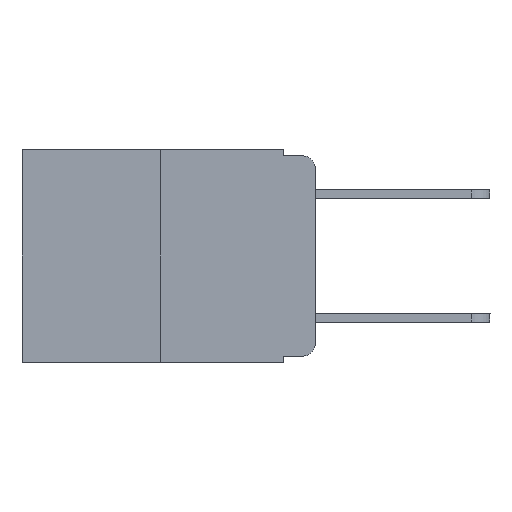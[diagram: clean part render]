
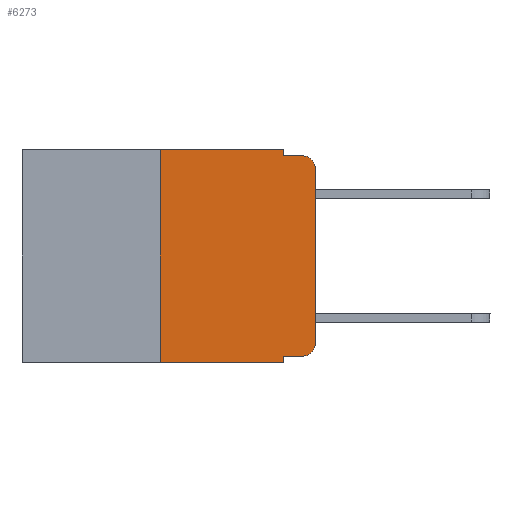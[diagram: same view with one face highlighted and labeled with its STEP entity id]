
A CAD part, left-side view. The second image highlights one B-rep face of the part: STEP entity #6273.
In plain terms, the highlighted planar face has unit normal (-1, 0, 0).
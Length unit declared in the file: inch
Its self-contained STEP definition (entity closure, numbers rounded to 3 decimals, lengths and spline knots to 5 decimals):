
#182 = CIRCLE ( 'NONE', #10225, 0.02 ) ;
#445 = CARTESIAN_POINT ( 'NONE',  ( 0., 0.051, -0.333 ) ) ;
#484 = VERTEX_POINT ( 'NONE', #7093 ) ;
#715 = CARTESIAN_POINT ( 'NONE',  ( 0., 0.051, 0. ) ) ;
#750 = ORIENTED_EDGE ( 'NONE', *, *, #6286, .T. ) ;
#757 = VERTEX_POINT ( 'NONE', #15017 ) ;
#823 = LINE ( 'NONE', #2420, #1748 ) ;
#1157 = DIRECTION ( 'NONE',  ( -1., 0., 0. ) ) ;
#1341 = ORIENTED_EDGE ( 'NONE', *, *, #10828, .T. ) ;
#1599 = ORIENTED_EDGE ( 'NONE', *, *, #10114, .F. ) ;
#1748 = VECTOR ( 'NONE', #13231, 39.37008 ) ;
#1976 = VECTOR ( 'NONE', #14798, 39.37008 ) ;
#2177 = CIRCLE ( 'NONE', #5035, 0.02 ) ;
#2183 = DIRECTION ( 'NONE',  ( 0., -1., 0. ) ) ;
#2420 = CARTESIAN_POINT ( 'NONE',  ( 0., 0.473, 0. ) ) ;
#2553 = LINE ( 'NONE', #9236, #14938 ) ;
#2560 = CARTESIAN_POINT ( 'NONE',  ( 0., 0., -0.03 ) ) ;
#2657 = VERTEX_POINT ( 'NONE', #14166 ) ;
#2874 = VERTEX_POINT ( 'NONE', #9908 ) ;
#3619 = ORIENTED_EDGE ( 'NONE', *, *, #7371, .F. ) ;
#3761 = CARTESIAN_POINT ( 'NONE',  ( 0., 0., 0. ) ) ;
#3786 = CARTESIAN_POINT ( 'NONE',  ( 0., 0.051, -0.01 ) ) ;
#4006 = CARTESIAN_POINT ( 'NONE',  ( 0., 0.051, -0.333 ) ) ;
#4274 = EDGE_LOOP ( 'NONE', ( #11995, #1341, #12284, #1599, #7026, #13450, #15163, #3619, #6871, #750 ) ) ;
#4278 = CARTESIAN_POINT ( 'NONE',  ( 0., 0.25, 0. ) ) ;
#4734 = PLANE ( 'NONE',  #6441 ) ;
#5035 = AXIS2_PLACEMENT_3D ( 'NONE', #5893, #5844, #8236 ) ;
#5484 = DIRECTION ( 'NONE',  ( 0., 0., 1. ) ) ;
#5844 = DIRECTION ( 'NONE',  ( -1., 0., 0. ) ) ;
#5893 = CARTESIAN_POINT ( 'NONE',  ( 0., 0.02, -0.313 ) ) ;
#5907 = LINE ( 'NONE', #445, #1976 ) ;
#6107 = VERTEX_POINT ( 'NONE', #4006 ) ;
#6273 = ADVANCED_FACE ( 'NONE', ( #10043 ), #4734, .F. ) ;
#6286 = EDGE_CURVE ( 'NONE', #10520, #2874, #2177, .T. ) ;
#6420 = LINE ( 'NONE', #3761, #13572 ) ;
#6441 = AXIS2_PLACEMENT_3D ( 'NONE', #13153, #12944, #12999 ) ;
#6871 = ORIENTED_EDGE ( 'NONE', *, *, #7789, .T. ) ;
#7026 = ORIENTED_EDGE ( 'NONE', *, *, #9501, .F. ) ;
#7093 = CARTESIAN_POINT ( 'NONE',  ( 0., 0.25, 0. ) ) ;
#7371 = EDGE_CURVE ( 'NONE', #6107, #757, #2553, .T. ) ;
#7789 = EDGE_CURVE ( 'NONE', #6107, #10520, #5907, .T. ) ;
#8124 = DIRECTION ( 'NONE',  ( 0., 0., -1. ) ) ;
#8236 = DIRECTION ( 'NONE',  ( 0., 0., -1. ) ) ;
#8783 = CARTESIAN_POINT ( 'NONE',  ( 0., 0.25, -0.343 ) ) ;
#9236 = CARTESIAN_POINT ( 'NONE',  ( 0., 0.051, 0. ) ) ;
#9501 = EDGE_CURVE ( 'NONE', #484, #14658, #823, .T. ) ;
#9786 = DIRECTION ( 'NONE',  ( 0., -1., 0. ) ) ;
#9908 = CARTESIAN_POINT ( 'NONE',  ( 0., 0., -0.313 ) ) ;
#9984 = EDGE_CURVE ( 'NONE', #15344, #484, #9996, .T. ) ;
#9996 = LINE ( 'NONE', #4278, #13950 ) ;
#10043 = FACE_OUTER_BOUND ( 'NONE', #4274, .T. ) ;
#10114 = EDGE_CURVE ( 'NONE', #14658, #11758, #15314, .T. ) ;
#10225 = AXIS2_PLACEMENT_3D ( 'NONE', #12977, #1157, #13076 ) ;
#10361 = EDGE_CURVE ( 'NONE', #15344, #757, #11421, .T. ) ;
#10520 = VERTEX_POINT ( 'NONE', #13720 ) ;
#10828 = EDGE_CURVE ( 'NONE', #14083, #2657, #182, .T. ) ;
#11421 = LINE ( 'NONE', #14139, #14247 ) ;
#11758 = VERTEX_POINT ( 'NONE', #13619 ) ;
#11995 = ORIENTED_EDGE ( 'NONE', *, *, #14094, .T. ) ;
#12224 = DIRECTION ( 'NONE',  ( 0., 0., 1. ) ) ;
#12284 = ORIENTED_EDGE ( 'NONE', *, *, #15110, .F. ) ;
#12944 = DIRECTION ( 'NONE',  ( 1., 0., 0. ) ) ;
#12977 = CARTESIAN_POINT ( 'NONE',  ( 0., 0.02, -0.03 ) ) ;
#12999 = DIRECTION ( 'NONE',  ( 0., 0., -1. ) ) ;
#13076 = DIRECTION ( 'NONE',  ( 0., 0., -1. ) ) ;
#13153 = CARTESIAN_POINT ( 'NONE',  ( 0., 0.473, 0. ) ) ;
#13231 = DIRECTION ( 'NONE',  ( 0., -1., 0. ) ) ;
#13363 = LINE ( 'NONE', #3786, #14661 ) ;
#13450 = ORIENTED_EDGE ( 'NONE', *, *, #9984, .F. ) ;
#13572 = VECTOR ( 'NONE', #12224, 39.37008 ) ;
#13614 = VECTOR ( 'NONE', #15286, 39.37008 ) ;
#13619 = CARTESIAN_POINT ( 'NONE',  ( 0., 0.051, -0.01 ) ) ;
#13720 = CARTESIAN_POINT ( 'NONE',  ( 0., 0.02, -0.333 ) ) ;
#13950 = VECTOR ( 'NONE', #5484, 39.37008 ) ;
#14083 = VERTEX_POINT ( 'NONE', #2560 ) ;
#14094 = EDGE_CURVE ( 'NONE', #2874, #14083, #6420, .T. ) ;
#14139 = CARTESIAN_POINT ( 'NONE',  ( 0., 0.473, -0.343 ) ) ;
#14166 = CARTESIAN_POINT ( 'NONE',  ( 0., 0.02, -0.01 ) ) ;
#14247 = VECTOR ( 'NONE', #2183, 39.37008 ) ;
#14658 = VERTEX_POINT ( 'NONE', #14659 ) ;
#14659 = CARTESIAN_POINT ( 'NONE',  ( 0., 0.051, 0. ) ) ;
#14661 = VECTOR ( 'NONE', #9786, 39.37008 ) ;
#14798 = DIRECTION ( 'NONE',  ( 0., -1., 0. ) ) ;
#14938 = VECTOR ( 'NONE', #8124, 39.37008 ) ;
#15017 = CARTESIAN_POINT ( 'NONE',  ( 0., 0.051, -0.343 ) ) ;
#15110 = EDGE_CURVE ( 'NONE', #11758, #2657, #13363, .T. ) ;
#15163 = ORIENTED_EDGE ( 'NONE', *, *, #10361, .T. ) ;
#15286 = DIRECTION ( 'NONE',  ( 0., 0., -1. ) ) ;
#15314 = LINE ( 'NONE', #715, #13614 ) ;
#15344 = VERTEX_POINT ( 'NONE', #8783 ) ;
